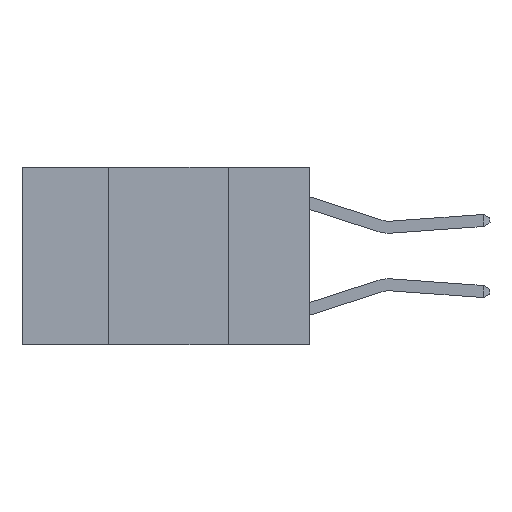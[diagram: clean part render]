
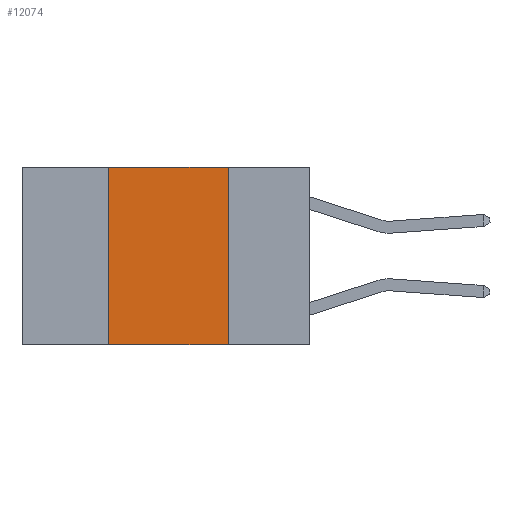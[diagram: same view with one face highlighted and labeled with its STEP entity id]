
A CAD part, left-side view. The second image highlights one B-rep face of the part: STEP entity #12074.
In plain terms, the highlighted planar face has unit normal (-1, 0, 0).
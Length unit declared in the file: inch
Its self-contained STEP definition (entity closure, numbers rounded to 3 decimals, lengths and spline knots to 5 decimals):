
#65 = CARTESIAN_POINT ( 'NONE',  ( 0., 0.6, 0. ) ) ;
#199 = VERTEX_POINT ( 'NONE', #19569 ) ;
#4227 = EDGE_CURVE ( 'NONE', #10179, #199, #7133, .T. ) ;
#4634 = FACE_OUTER_BOUND ( 'NONE', #18716, .T. ) ;
#4789 = DIRECTION ( 'NONE',  ( 0., -1., 0. ) ) ;
#5058 = ORIENTED_EDGE ( 'NONE', *, *, #25550, .T. ) ;
#6951 = CARTESIAN_POINT ( 'NONE',  ( 0., 0.42, 0. ) ) ;
#7008 = DIRECTION ( 'NONE',  ( 1., 0., 0. ) ) ;
#7133 = LINE ( 'NONE', #65, #24013 ) ;
#7149 = DIRECTION ( 'NONE',  ( 0., -1., 0. ) ) ;
#7585 = ORIENTED_EDGE ( 'NONE', *, *, #8039, .F. ) ;
#8039 = EDGE_CURVE ( 'NONE', #199, #21650, #9426, .T. ) ;
#8390 = CARTESIAN_POINT ( 'NONE',  ( 0., 0.17, 0. ) ) ;
#9426 = LINE ( 'NONE', #8390, #27029 ) ;
#10179 = VERTEX_POINT ( 'NONE', #6951 ) ;
#12074 = ADVANCED_FACE ( 'NONE', ( #4634 ), #27608, .F. ) ;
#12322 = VECTOR ( 'NONE', #4789, 39.37008 ) ;
#12837 = CARTESIAN_POINT ( 'NONE',  ( 0., 0.42, 0. ) ) ;
#14788 = EDGE_CURVE ( 'NONE', #19048, #10179, #17454, .T. ) ;
#15154 = DIRECTION ( 'NONE',  ( 0., 0., 1. ) ) ;
#15155 = ORIENTED_EDGE ( 'NONE', *, *, #4227, .F. ) ;
#15877 = ORIENTED_EDGE ( 'NONE', *, *, #14788, .F. ) ;
#16277 = CARTESIAN_POINT ( 'NONE',  ( 0., 0.6, -0.37 ) ) ;
#17454 = LINE ( 'NONE', #12837, #23543 ) ;
#17730 = LINE ( 'NONE', #16277, #12322 ) ;
#18716 = EDGE_LOOP ( 'NONE', ( #7585, #15155, #15877, #5058 ) ) ;
#19048 = VERTEX_POINT ( 'NONE', #23029 ) ;
#19569 = CARTESIAN_POINT ( 'NONE',  ( 0., 0.17, 0. ) ) ;
#21650 = VERTEX_POINT ( 'NONE', #28200 ) ;
#22120 = DIRECTION ( 'NONE',  ( 0., 0., -1. ) ) ;
#22637 = AXIS2_PLACEMENT_3D ( 'NONE', #25150, #7008, #23060 ) ;
#23029 = CARTESIAN_POINT ( 'NONE',  ( 0., 0.42, -0.37 ) ) ;
#23060 = DIRECTION ( 'NONE',  ( 0., 0., -1. ) ) ;
#23543 = VECTOR ( 'NONE', #15154, 39.37008 ) ;
#24013 = VECTOR ( 'NONE', #7149, 39.37008 ) ;
#25150 = CARTESIAN_POINT ( 'NONE',  ( 0., 0.6, 0. ) ) ;
#25550 = EDGE_CURVE ( 'NONE', #19048, #21650, #17730, .T. ) ;
#27029 = VECTOR ( 'NONE', #22120, 39.37008 ) ;
#27608 = PLANE ( 'NONE',  #22637 ) ;
#28200 = CARTESIAN_POINT ( 'NONE',  ( 0., 0.17, -0.37 ) ) ;
